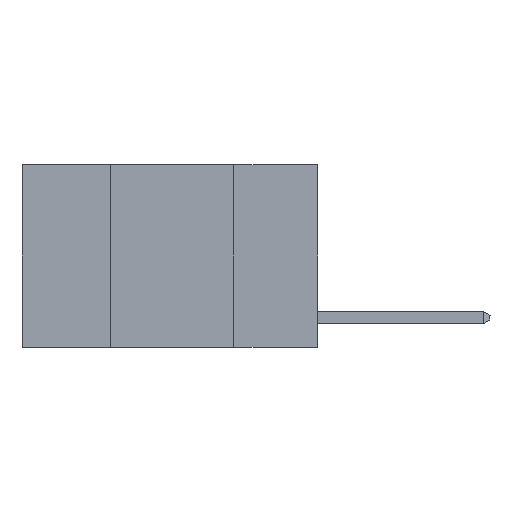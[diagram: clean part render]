
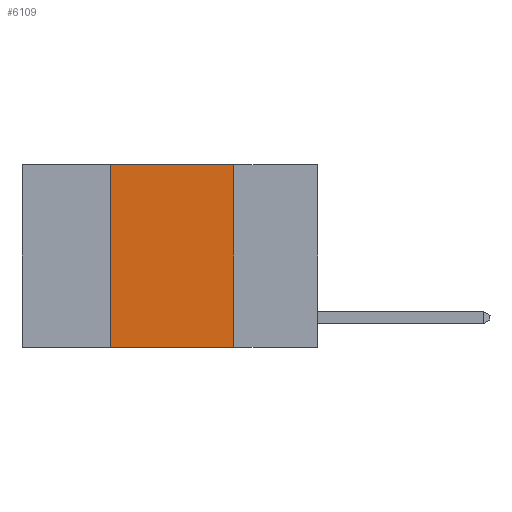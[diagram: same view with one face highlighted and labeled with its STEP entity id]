
A CAD part, left-side view. The second image highlights one B-rep face of the part: STEP entity #6109.
In plain terms, the highlighted planar face has unit normal (-1, 0, 0).
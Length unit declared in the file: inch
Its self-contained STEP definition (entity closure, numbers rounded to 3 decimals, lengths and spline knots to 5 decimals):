
#432 = VECTOR ( 'NONE', #9067, 39.37008 ) ;
#886 = CARTESIAN_POINT ( 'NONE',  ( 0., 0.17, 0. ) ) ;
#1782 = EDGE_CURVE ( 'NONE', #5801, #8173, #5294, .T. ) ;
#2583 = DIRECTION ( 'NONE',  ( 1., 0., 0. ) ) ;
#3021 = EDGE_CURVE ( 'NONE', #5801, #6911, #13040, .T. ) ;
#4107 = ORIENTED_EDGE ( 'NONE', *, *, #1782, .T. ) ;
#4304 = CARTESIAN_POINT ( 'NONE',  ( 0., 0.17, 0. ) ) ;
#4494 = AXIS2_PLACEMENT_3D ( 'NONE', #11572, #2583, #10470 ) ;
#5056 = EDGE_LOOP ( 'NONE', ( #5997, #11225, #13973, #4107 ) ) ;
#5294 = LINE ( 'NONE', #7378, #12383 ) ;
#5632 = EDGE_CURVE ( 'NONE', #9340, #8173, #12600, .T. ) ;
#5766 = EDGE_CURVE ( 'NONE', #6911, #9340, #6223, .T. ) ;
#5801 = VERTEX_POINT ( 'NONE', #7017 ) ;
#5997 = ORIENTED_EDGE ( 'NONE', *, *, #5632, .F. ) ;
#6109 = ADVANCED_FACE ( 'NONE', ( #7491 ), #8202, .F. ) ;
#6223 = LINE ( 'NONE', #12300, #432 ) ;
#6871 = DIRECTION ( 'NONE',  ( 0., 0., -1. ) ) ;
#6911 = VERTEX_POINT ( 'NONE', #11241 ) ;
#7017 = CARTESIAN_POINT ( 'NONE',  ( 0., 0.42, -0.37 ) ) ;
#7378 = CARTESIAN_POINT ( 'NONE',  ( 0., 0.6, -0.37 ) ) ;
#7491 = FACE_OUTER_BOUND ( 'NONE', #5056, .T. ) ;
#8173 = VERTEX_POINT ( 'NONE', #13273 ) ;
#8202 = PLANE ( 'NONE',  #4494 ) ;
#8255 = VECTOR ( 'NONE', #8925, 39.37008 ) ;
#8378 = VECTOR ( 'NONE', #6871, 39.37008 ) ;
#8503 = DIRECTION ( 'NONE',  ( 0., -1., 0. ) ) ;
#8925 = DIRECTION ( 'NONE',  ( 0., 0., 1. ) ) ;
#9067 = DIRECTION ( 'NONE',  ( 0., -1., 0. ) ) ;
#9340 = VERTEX_POINT ( 'NONE', #4304 ) ;
#10470 = DIRECTION ( 'NONE',  ( 0., 0., -1. ) ) ;
#11225 = ORIENTED_EDGE ( 'NONE', *, *, #5766, .F. ) ;
#11241 = CARTESIAN_POINT ( 'NONE',  ( 0., 0.42, 0. ) ) ;
#11572 = CARTESIAN_POINT ( 'NONE',  ( 0., 0.6, 0. ) ) ;
#12158 = CARTESIAN_POINT ( 'NONE',  ( 0., 0.42, 0. ) ) ;
#12300 = CARTESIAN_POINT ( 'NONE',  ( 0., 0.6, 0. ) ) ;
#12383 = VECTOR ( 'NONE', #8503, 39.37008 ) ;
#12600 = LINE ( 'NONE', #886, #8378 ) ;
#13040 = LINE ( 'NONE', #12158, #8255 ) ;
#13273 = CARTESIAN_POINT ( 'NONE',  ( 0., 0.17, -0.37 ) ) ;
#13973 = ORIENTED_EDGE ( 'NONE', *, *, #3021, .F. ) ;
